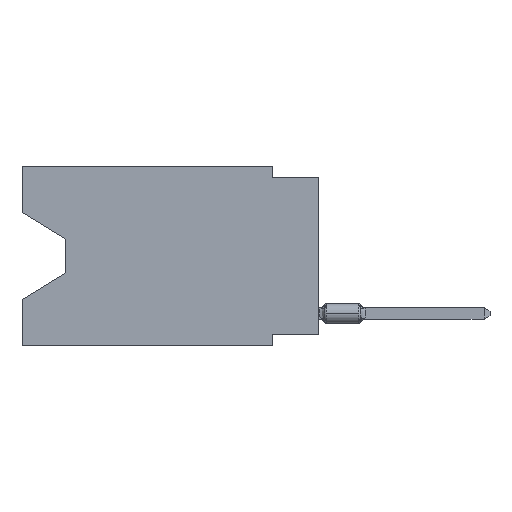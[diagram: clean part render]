
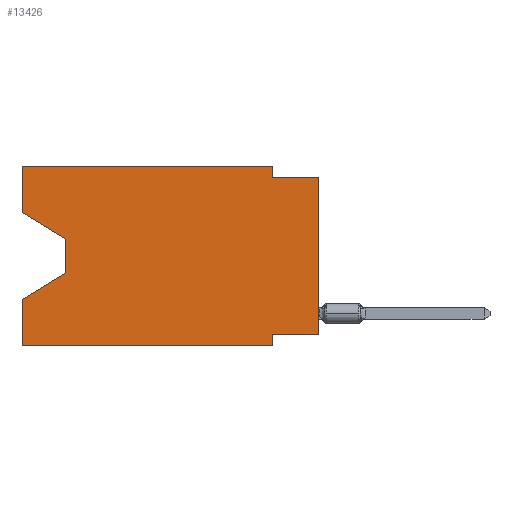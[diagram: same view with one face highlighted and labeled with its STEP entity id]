
A CAD part, left-side view. The second image highlights one B-rep face of the part: STEP entity #13426.
In plain terms, the highlighted planar face has unit normal (-1, 0, 0).
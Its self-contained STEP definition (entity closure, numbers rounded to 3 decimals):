
#73 = EDGE_LOOP ( 'NONE', ( #2701, #15213, #14170, #15176, #8682, #2969, #5076, #13410, #3907, #11868, #2363, #8598 ) ) ;
#316 = CARTESIAN_POINT ( 'NONE',  ( 0., 16.383, -2.546 ) ) ;
#485 = CARTESIAN_POINT ( 'NONE',  ( 0., 13.97, -5.893 ) ) ;
#743 = CARTESIAN_POINT ( 'NONE',  ( 0., 2.54, -9.906 ) ) ;
#987 = DIRECTION ( 'NONE',  ( 0., -1., 0. ) ) ;
#1068 = LINE ( 'NONE', #10494, #2439 ) ;
#1092 = CARTESIAN_POINT ( 'NONE',  ( 0., 2.54, 0. ) ) ;
#1253 = DIRECTION ( 'NONE',  ( 0., 0., -1. ) ) ;
#1499 = CARTESIAN_POINT ( 'NONE',  ( 0., 13.97, -5.893 ) ) ;
#1629 = VECTOR ( 'NONE', #9888, 1000. ) ;
#1770 = CARTESIAN_POINT ( 'NONE',  ( 0., 2.54, 0. ) ) ;
#1979 = CARTESIAN_POINT ( 'NONE',  ( 0., 2.54, -9.906 ) ) ;
#2101 = VERTEX_POINT ( 'NONE', #8987 ) ;
#2363 = ORIENTED_EDGE ( 'NONE', *, *, #10882, .F. ) ;
#2439 = VECTOR ( 'NONE', #987, 1000. ) ;
#2539 = CARTESIAN_POINT ( 'NONE',  ( 0., 0., -0.635 ) ) ;
#2701 = ORIENTED_EDGE ( 'NONE', *, *, #10063, .T. ) ;
#2736 = VERTEX_POINT ( 'NONE', #485 ) ;
#2969 = ORIENTED_EDGE ( 'NONE', *, *, #6849, .F. ) ;
#3373 = DIRECTION ( 'NONE',  ( 0., 0., -1. ) ) ;
#3378 = CARTESIAN_POINT ( 'NONE',  ( 0., 13.97, -4.013 ) ) ;
#3525 = CARTESIAN_POINT ( 'NONE',  ( 0., 2.54, -9.271 ) ) ;
#3612 = CARTESIAN_POINT ( 'NONE',  ( 0., 16.383, 0. ) ) ;
#3907 = ORIENTED_EDGE ( 'NONE', *, *, #6246, .F. ) ;
#4281 = VERTEX_POINT ( 'NONE', #1770 ) ;
#4415 = VECTOR ( 'NONE', #1253, 1000. ) ;
#4709 = LINE ( 'NONE', #3378, #4736 ) ;
#4736 = VECTOR ( 'NONE', #8095, 1000. ) ;
#4840 = VECTOR ( 'NONE', #10919, 1000. ) ;
#4969 = LINE ( 'NONE', #14516, #15414 ) ;
#5047 = LINE ( 'NONE', #6146, #6770 ) ;
#5051 = VECTOR ( 'NONE', #7303, 1000. ) ;
#5076 = ORIENTED_EDGE ( 'NONE', *, *, #11412, .F. ) ;
#5101 = DIRECTION ( 'NONE',  ( 0., -1., 0. ) ) ;
#5208 = DIRECTION ( 'NONE',  ( 0., 0., 1. ) ) ;
#5513 = LINE ( 'NONE', #743, #6983 ) ;
#5680 = VERTEX_POINT ( 'NONE', #5814 ) ;
#5724 = CARTESIAN_POINT ( 'NONE',  ( 0., 16.383, 0. ) ) ;
#5730 = VERTEX_POINT ( 'NONE', #9849 ) ;
#5814 = CARTESIAN_POINT ( 'NONE',  ( 0., 2.54, -0.635 ) ) ;
#5881 = FACE_OUTER_BOUND ( 'NONE', #73, .T. ) ;
#5935 = CARTESIAN_POINT ( 'NONE',  ( 0., 16.383, -2.546 ) ) ;
#6135 = CARTESIAN_POINT ( 'NONE',  ( 0., 16.383, 0. ) ) ;
#6146 = CARTESIAN_POINT ( 'NONE',  ( 0., 16.383, 0. ) ) ;
#6182 = VERTEX_POINT ( 'NONE', #3525 ) ;
#6246 = EDGE_CURVE ( 'NONE', #5680, #12216, #8479, .T. ) ;
#6568 = VERTEX_POINT ( 'NONE', #1979 ) ;
#6645 = LINE ( 'NONE', #11228, #12102 ) ;
#6770 = VECTOR ( 'NONE', #14664, 1000. ) ;
#6789 = CARTESIAN_POINT ( 'NONE',  ( 0., 0., -9.271 ) ) ;
#6849 = EDGE_CURVE ( 'NONE', #6182, #6568, #5513, .T. ) ;
#6853 = CARTESIAN_POINT ( 'NONE',  ( 0., 0., -0.635 ) ) ;
#6964 = VECTOR ( 'NONE', #9215, 1000. ) ;
#6983 = VECTOR ( 'NONE', #7726, 1000. ) ;
#7002 = EDGE_CURVE ( 'NONE', #2101, #2736, #4709, .T. ) ;
#7201 = LINE ( 'NONE', #316, #4840 ) ;
#7303 = DIRECTION ( 'NONE',  ( 0., -1., 0. ) ) ;
#7726 = DIRECTION ( 'NONE',  ( 0., 0., -1. ) ) ;
#7842 = AXIS2_PLACEMENT_3D ( 'NONE', #5724, #12971, #3373 ) ;
#7882 = CARTESIAN_POINT ( 'NONE',  ( 0., 16.383, -7.36 ) ) ;
#7942 = PLANE ( 'NONE',  #7842 ) ;
#7991 = EDGE_CURVE ( 'NONE', #5730, #12216, #6645, .T. ) ;
#8029 = VECTOR ( 'NONE', #5101, 1000. ) ;
#8095 = DIRECTION ( 'NONE',  ( 0., 0., -1. ) ) ;
#8446 = EDGE_CURVE ( 'NONE', #10925, #12149, #4969, .T. ) ;
#8479 = LINE ( 'NONE', #2539, #5051 ) ;
#8598 = ORIENTED_EDGE ( 'NONE', *, *, #11697, .F. ) ;
#8682 = ORIENTED_EDGE ( 'NONE', *, *, #15545, .T. ) ;
#8987 = CARTESIAN_POINT ( 'NONE',  ( 0., 13.97, -4.013 ) ) ;
#9032 = EDGE_CURVE ( 'NONE', #2736, #12149, #14773, .T. ) ;
#9215 = DIRECTION ( 'NONE',  ( 0., 1., 0. ) ) ;
#9808 = VERTEX_POINT ( 'NONE', #6135 ) ;
#9849 = CARTESIAN_POINT ( 'NONE',  ( 0., 0., -9.271 ) ) ;
#9888 = DIRECTION ( 'NONE',  ( 0., 0.855, -0.519 ) ) ;
#10039 = VERTEX_POINT ( 'NONE', #5935 ) ;
#10063 = EDGE_CURVE ( 'NONE', #10039, #2101, #7201, .T. ) ;
#10494 = CARTESIAN_POINT ( 'NONE',  ( 0., 16.383, -9.906 ) ) ;
#10882 = EDGE_CURVE ( 'NONE', #9808, #4281, #12095, .T. ) ;
#10919 = DIRECTION ( 'NONE',  ( 0., -0.855, -0.519 ) ) ;
#10925 = VERTEX_POINT ( 'NONE', #12017 ) ;
#11150 = DIRECTION ( 'NONE',  ( 0., 0., 1. ) ) ;
#11228 = CARTESIAN_POINT ( 'NONE',  ( 0., 0., 0. ) ) ;
#11412 = EDGE_CURVE ( 'NONE', #5730, #6182, #12689, .T. ) ;
#11697 = EDGE_CURVE ( 'NONE', #10039, #9808, #5047, .T. ) ;
#11868 = ORIENTED_EDGE ( 'NONE', *, *, #15122, .F. ) ;
#12017 = CARTESIAN_POINT ( 'NONE',  ( 0., 16.383, -9.906 ) ) ;
#12095 = LINE ( 'NONE', #3612, #8029 ) ;
#12102 = VECTOR ( 'NONE', #11150, 1000. ) ;
#12149 = VERTEX_POINT ( 'NONE', #7882 ) ;
#12216 = VERTEX_POINT ( 'NONE', #6853 ) ;
#12689 = LINE ( 'NONE', #6789, #6964 ) ;
#12971 = DIRECTION ( 'NONE',  ( 1., 0., 0. ) ) ;
#13021 = LINE ( 'NONE', #1092, #4415 ) ;
#13410 = ORIENTED_EDGE ( 'NONE', *, *, #7991, .T. ) ;
#13426 = ADVANCED_FACE ( 'NONE', ( #5881 ), #7942, .F. ) ;
#14170 = ORIENTED_EDGE ( 'NONE', *, *, #9032, .T. ) ;
#14516 = CARTESIAN_POINT ( 'NONE',  ( 0., 16.383, 0. ) ) ;
#14664 = DIRECTION ( 'NONE',  ( 0., 0., 1. ) ) ;
#14773 = LINE ( 'NONE', #1499, #1629 ) ;
#15122 = EDGE_CURVE ( 'NONE', #4281, #5680, #13021, .T. ) ;
#15176 = ORIENTED_EDGE ( 'NONE', *, *, #8446, .F. ) ;
#15213 = ORIENTED_EDGE ( 'NONE', *, *, #7002, .T. ) ;
#15414 = VECTOR ( 'NONE', #5208, 1000. ) ;
#15545 = EDGE_CURVE ( 'NONE', #10925, #6568, #1068, .T. ) ;
